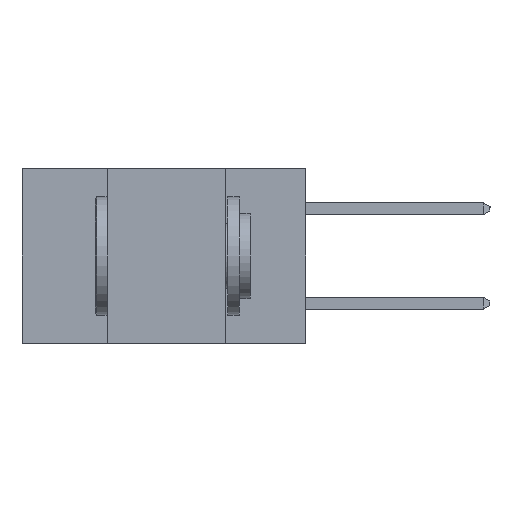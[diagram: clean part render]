
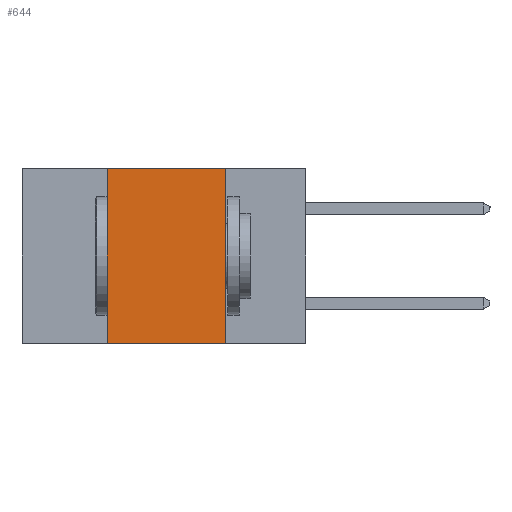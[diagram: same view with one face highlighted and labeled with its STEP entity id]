
A CAD part, left-side view. The second image highlights one B-rep face of the part: STEP entity #644.
In plain terms, the highlighted planar face has unit normal (-1, 0, 0).
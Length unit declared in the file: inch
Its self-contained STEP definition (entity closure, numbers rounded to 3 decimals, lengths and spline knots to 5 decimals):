
#70 = FACE_OUTER_BOUND ( 'NONE', #11113, .T. ) ;
#152 = LINE ( 'NONE', #2267, #6811 ) ;
#644 = ADVANCED_FACE ( 'NONE', ( #70 ), #8323, .F. ) ;
#1356 = ORIENTED_EDGE ( 'NONE', *, *, #2288, .F. ) ;
#1653 = CARTESIAN_POINT ( 'NONE',  ( 0., 0.6, 0. ) ) ;
#2009 = CARTESIAN_POINT ( 'NONE',  ( 0., 0.17, -0.37 ) ) ;
#2136 = ORIENTED_EDGE ( 'NONE', *, *, #4510, .F. ) ;
#2160 = ORIENTED_EDGE ( 'NONE', *, *, #7158, .F. ) ;
#2267 = CARTESIAN_POINT ( 'NONE',  ( 0., 0.6, -0.37 ) ) ;
#2288 = EDGE_CURVE ( 'NONE', #3223, #2387, #2537, .T. ) ;
#2370 = VECTOR ( 'NONE', #11292, 39.37008 ) ;
#2387 = VERTEX_POINT ( 'NONE', #4661 ) ;
#2478 = DIRECTION ( 'NONE',  ( 1., 0., 0. ) ) ;
#2537 = LINE ( 'NONE', #10326, #2370 ) ;
#2899 = CARTESIAN_POINT ( 'NONE',  ( 0., 0.17, 0. ) ) ;
#3223 = VERTEX_POINT ( 'NONE', #4745 ) ;
#3750 = AXIS2_PLACEMENT_3D ( 'NONE', #7856, #2478, #12215 ) ;
#3832 = VECTOR ( 'NONE', #11330, 39.37008 ) ;
#4357 = ORIENTED_EDGE ( 'NONE', *, *, #8673, .T. ) ;
#4510 = EDGE_CURVE ( 'NONE', #2387, #6946, #4905, .T. ) ;
#4661 = CARTESIAN_POINT ( 'NONE',  ( 0., 0.42, 0. ) ) ;
#4745 = CARTESIAN_POINT ( 'NONE',  ( 0., 0.42, -0.37 ) ) ;
#4905 = LINE ( 'NONE', #1653, #3832 ) ;
#5480 = VECTOR ( 'NONE', #6511, 39.37008 ) ;
#6511 = DIRECTION ( 'NONE',  ( 0., 0., -1. ) ) ;
#6811 = VECTOR ( 'NONE', #13233, 39.37008 ) ;
#6946 = VERTEX_POINT ( 'NONE', #2899 ) ;
#7158 = EDGE_CURVE ( 'NONE', #6946, #11984, #9694, .T. ) ;
#7856 = CARTESIAN_POINT ( 'NONE',  ( 0., 0.6, 0. ) ) ;
#8323 = PLANE ( 'NONE',  #3750 ) ;
#8673 = EDGE_CURVE ( 'NONE', #3223, #11984, #152, .T. ) ;
#9694 = LINE ( 'NONE', #9758, #5480 ) ;
#9758 = CARTESIAN_POINT ( 'NONE',  ( 0., 0.17, -0.37 ) ) ;
#10326 = CARTESIAN_POINT ( 'NONE',  ( 0., 0.42, -0.37 ) ) ;
#11113 = EDGE_LOOP ( 'NONE', ( #2160, #2136, #1356, #4357 ) ) ;
#11292 = DIRECTION ( 'NONE',  ( 0., 0., 1. ) ) ;
#11330 = DIRECTION ( 'NONE',  ( 0., -1., 0. ) ) ;
#11984 = VERTEX_POINT ( 'NONE', #2009 ) ;
#12215 = DIRECTION ( 'NONE',  ( 0., 0., -1. ) ) ;
#13233 = DIRECTION ( 'NONE',  ( 0., -1., 0. ) ) ;
